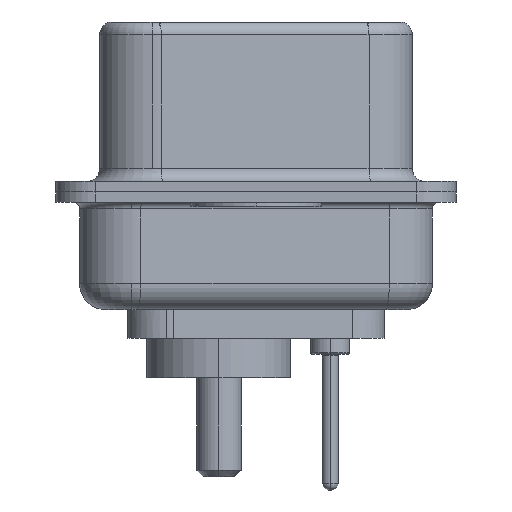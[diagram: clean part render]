
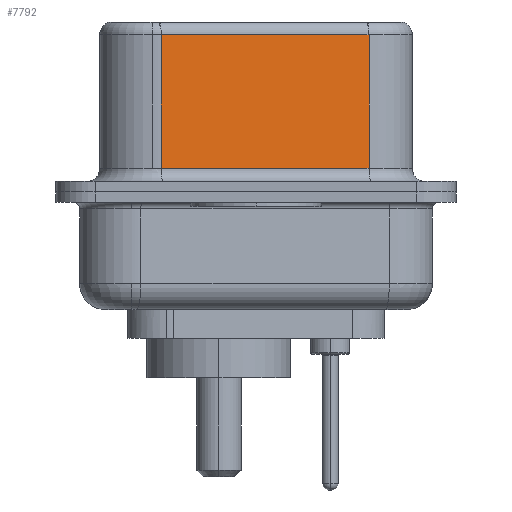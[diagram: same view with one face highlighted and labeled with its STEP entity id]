
A CAD part, left-side view. The second image highlights one B-rep face of the part: STEP entity #7792.
In plain terms, the highlighted planar face has unit normal (-0.985, -0.174, 0).
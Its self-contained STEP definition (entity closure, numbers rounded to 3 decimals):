
#95 = EDGE_CURVE ( 'NONE', #194, #12387, #8294, .T. ) ;
#194 = VERTEX_POINT ( 'NONE', #3883 ) ;
#575 = AXIS2_PLACEMENT_3D ( 'NONE', #9640, #11795, #2512 ) ;
#1074 = EDGE_LOOP ( 'NONE', ( #16354, #15583, #3825, #16626 ) ) ;
#1781 = DIRECTION ( 'NONE',  ( -0.174, 0.985, 0. ) ) ;
#2512 = DIRECTION ( 'NONE',  ( -0.174, 0.985, 0. ) ) ;
#3825 = ORIENTED_EDGE ( 'NONE', *, *, #8500, .T. ) ;
#3883 = CARTESIAN_POINT ( 'NONE',  ( 3.73, 3.628, 0.9 ) ) ;
#4350 = LINE ( 'NONE', #15216, #14378 ) ;
#4683 = VERTEX_POINT ( 'NONE', #7874 ) ;
#4703 = CARTESIAN_POINT ( 'NONE',  ( 5.132, -4.322, 6.02 ) ) ;
#7587 = CARTESIAN_POINT ( 'NONE',  ( 3.73, 3.628, 6.02 ) ) ;
#7693 = VECTOR ( 'NONE', #1781, 1000. ) ;
#7792 = ADVANCED_FACE ( 'NONE', ( #15115 ), #16034, .F. ) ;
#7874 = CARTESIAN_POINT ( 'NONE',  ( 5.132, -4.322, 6.02 ) ) ;
#8035 = LINE ( 'NONE', #16926, #11578 ) ;
#8294 = LINE ( 'NONE', #11875, #15793 ) ;
#8500 = EDGE_CURVE ( 'NONE', #15565, #194, #4350, .T. ) ;
#9265 = CARTESIAN_POINT ( 'NONE',  ( 5.132, -4.322, 0.9 ) ) ;
#9640 = CARTESIAN_POINT ( 'NONE',  ( 5.132, -4.322, 6.52 ) ) ;
#11262 = EDGE_CURVE ( 'NONE', #4683, #15565, #15676, .T. ) ;
#11578 = VECTOR ( 'NONE', #12534, 1000. ) ;
#11795 = DIRECTION ( 'NONE',  ( 0.985, 0.174, 0. ) ) ;
#11875 = CARTESIAN_POINT ( 'NONE',  ( 5.132, -4.322, 0.9 ) ) ;
#12387 = VERTEX_POINT ( 'NONE', #9265 ) ;
#12534 = DIRECTION ( 'NONE',  ( 0., 0., -1. ) ) ;
#14378 = VECTOR ( 'NONE', #18093, 1000. ) ;
#15115 = FACE_OUTER_BOUND ( 'NONE', #1074, .T. ) ;
#15216 = CARTESIAN_POINT ( 'NONE',  ( 3.73, 3.628, 6.52 ) ) ;
#15565 = VERTEX_POINT ( 'NONE', #7587 ) ;
#15583 = ORIENTED_EDGE ( 'NONE', *, *, #11262, .T. ) ;
#15676 = LINE ( 'NONE', #4703, #7693 ) ;
#15712 = DIRECTION ( 'NONE',  ( 0.174, -0.985, 0. ) ) ;
#15793 = VECTOR ( 'NONE', #15712, 1000. ) ;
#16034 = PLANE ( 'NONE',  #575 ) ;
#16354 = ORIENTED_EDGE ( 'NONE', *, *, #16378, .F. ) ;
#16378 = EDGE_CURVE ( 'NONE', #4683, #12387, #8035, .T. ) ;
#16626 = ORIENTED_EDGE ( 'NONE', *, *, #95, .T. ) ;
#16926 = CARTESIAN_POINT ( 'NONE',  ( 5.132, -4.322, 6.52 ) ) ;
#18093 = DIRECTION ( 'NONE',  ( 0., 0., -1. ) ) ;
